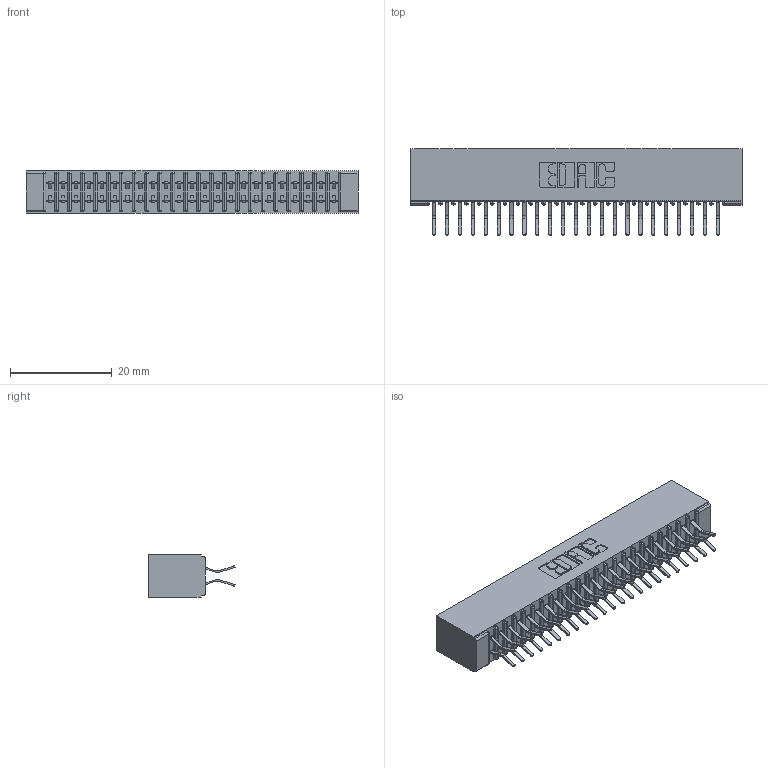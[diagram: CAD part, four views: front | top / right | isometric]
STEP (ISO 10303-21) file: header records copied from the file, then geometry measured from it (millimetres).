
FILE_DESCRIPTION (( 'STEP AP203' ), '1' );
FILE_NAME ('391-046-556-201.STEP', '2018-08-09T03:33:51', ( '' ), ( '' ), 'SwSTEP 2.0', 'SolidWorks 2016', '' );
FILE_SCHEMA (( 'CONFIG_CONTROL_DESIGN' ));
Length unit declared in the file: inch
Products named in the file (3): 341 Part_No Mounting Lugs; 341-292-001_341-292-156; 391-046-556-201
Assembly tree (47 placements, depth 2):
  391-046-556-201
    341 Part_No Mounting Lugs
    341-292-001_341-292-156  x46
Bounding box: 65.41 x 17.07 x 8.38 mm (x, y, z)
Volume: 3864.3 mm3; surface area: 8891.6 mm2
Topology: 47 solids, 47 shells, 3328 faces, 9653 edges, 6262 vertices
Faces by surface type: plane 1904, cylinder 1332, sphere 48, torus 44
Entity records: 30228 total; most frequent: CARTESIAN_POINT 5025, ORIENTED_EDGE 4990, DIRECTION 4893, EDGE_CURVE 2495, LINE 1993, VECTOR 1993, VERTEX_POINT 1582, AXIS2_PLACEMENT_3D 1450
